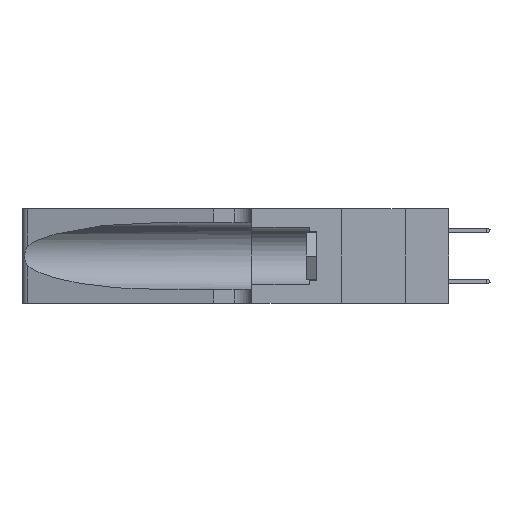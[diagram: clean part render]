
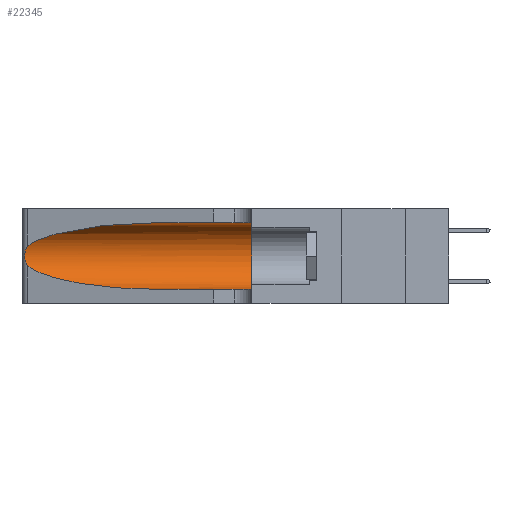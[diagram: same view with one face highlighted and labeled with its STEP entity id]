
A CAD part, left-side view. The second image highlights one B-rep face of the part: STEP entity #22345.
In plain terms, the highlighted cylindrical face has radius 3.308 mm (diameter 6.617 mm), a partial arc.
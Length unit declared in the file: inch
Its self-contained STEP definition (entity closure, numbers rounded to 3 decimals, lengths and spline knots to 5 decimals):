
#744 = CIRCLE ( 'NONE', #11254, 0.13025 ) ;
#951 = CARTESIAN_POINT ( 'NONE',  ( 0.1305, 0.35, 0.31525 ) ) ;
#1829 = ORIENTED_EDGE ( 'NONE', *, *, #18322, .F. ) ;
#2564 = CARTESIAN_POINT ( 'NONE',  ( 0.26017, 1.23833, 0.17102 ) ) ;
#2788 = LINE ( 'NONE', #3712, #29474 ) ;
#2856 = ORIENTED_EDGE ( 'NONE', *, *, #6467, .T. ) ;
#3712 = CARTESIAN_POINT ( 'NONE',  ( 0.1305, 1.61858, 0.05475 ) ) ;
#3921 = CARTESIAN_POINT ( 'NONE',  ( 0.26075, 1.23896, 0.19203 ) ) ;
#4350 = VERTEX_POINT ( 'NONE', #24508 ) ;
#4624 = B_SPLINE_CURVE_WITH_KNOTS ( 'NONE', 3,
 ( #23234, #12835, #28358, #12942, #30916, #15528, #3921, #18099, #2564, #20716, #5181, #23336, #7820, #25904 ),
 .UNSPECIFIED., .F., .F.,
 ( 4, 2, 2, 2, 2, 2, 4 ),
 ( 0., 0.00027, 0.00053, 0.00107, 0.0016, 0.00187, 0.00214 ),
 .UNSPECIFIED. ) ;
#4976 = CARTESIAN_POINT ( 'NONE',  ( 0.1305, 0.35, 0.185 ) ) ;
#5181 = CARTESIAN_POINT ( 'NONE',  ( 0.25789, 1.23486, 0.15765 ) ) ;
#6467 = EDGE_CURVE ( 'NONE', #20797, #4350, #19176, .T. ) ;
#6964 = CARTESIAN_POINT ( 'NONE',  ( 0.18966, 0.96281, 0.31525 ) ) ;
#7266 = EDGE_LOOP ( 'NONE', ( #2856, #14822, #15873, #10875, #1829, #7326 ) ) ;
#7326 = ORIENTED_EDGE ( 'NONE', *, *, #24627, .F. ) ;
#7609 = DIRECTION ( 'NONE',  ( 0., 0., 1. ) ) ;
#7820 = CARTESIAN_POINT ( 'NONE',  ( 0.25555, 1.22993, 0.14849 ) ) ;
#7839 = DIRECTION ( 'NONE',  ( 0., 0., -1. ) ) ;
#8406 = CARTESIAN_POINT ( 'NONE',  ( 0.18966, 0.96281, 0.05475 ) ) ;
#9448 = VECTOR ( 'NONE', #11316, 39.37008 ) ;
#10678 =( BOUNDED_CURVE ( )  B_SPLINE_CURVE ( 3, ( #18705, #10918, #8406, #26484 ),
 .UNSPECIFIED., .F., .T. ) 
 B_SPLINE_CURVE_WITH_KNOTS ( ( 4, 4 ),
 ( 3.44316, 4.71239 ),
 .UNSPECIFIED. ) 
 CURVE ( )  GEOMETRIC_REPRESENTATION_ITEM ( )  RATIONAL_B_SPLINE_CURVE ( ( 1., 0.87, 0.87, 1. ) ) 
 REPRESENTATION_ITEM ( '' )  );
#10875 = ORIENTED_EDGE ( 'NONE', *, *, #18711, .T. ) ;
#10918 = CARTESIAN_POINT ( 'NONE',  ( 0.2373, 1.15595, 0.08982 ) ) ;
#11254 = AXIS2_PLACEMENT_3D ( 'NONE', #4976, #23130, #7609 ) ;
#11316 = DIRECTION ( 'NONE',  ( 0., -1., 0. ) ) ;
#11328 = VERTEX_POINT ( 'NONE', #19131 ) ;
#12050 = FACE_OUTER_BOUND ( 'NONE', #7266, .T. ) ;
#12204 = CARTESIAN_POINT ( 'NONE',  ( 0.25487, 1.22718, 0.22369 ) ) ;
#12835 = CARTESIAN_POINT ( 'NONE',  ( 0.25555, 1.22994, 0.2215 ) ) ;
#12942 = CARTESIAN_POINT ( 'NONE',  ( 0.25787, 1.23484, 0.2124 ) ) ;
#14822 = ORIENTED_EDGE ( 'NONE', *, *, #30106, .T. ) ;
#15528 = CARTESIAN_POINT ( 'NONE',  ( 0.26018, 1.23835, 0.19895 ) ) ;
#15544 = DIRECTION ( 'NONE',  ( 0., -1., 0. ) ) ;
#15873 = ORIENTED_EDGE ( 'NONE', *, *, #29612, .T. ) ;
#18099 = CARTESIAN_POINT ( 'NONE',  ( 0.26075, 1.23896, 0.178 ) ) ;
#18322 = EDGE_CURVE ( 'NONE', #29056, #11328, #744, .T. ) ;
#18705 = CARTESIAN_POINT ( 'NONE',  ( 0.25487, 1.22718, 0.14631 ) ) ;
#18711 = EDGE_CURVE ( 'NONE', #31708, #11328, #2788, .T. ) ;
#18975 = CARTESIAN_POINT ( 'NONE',  ( 0.1305, 1.61858, 0.31525 ) ) ;
#19131 = CARTESIAN_POINT ( 'NONE',  ( 0.1305, 0.35, 0.05475 ) ) ;
#19176 =( BOUNDED_CURVE ( )  B_SPLINE_CURVE ( 3, ( #22364, #6964, #27633, #12204 ),
 .UNSPECIFIED., .F., .F. ) 
 B_SPLINE_CURVE_WITH_KNOTS ( ( 4, 4 ),
 ( 1.5708, 2.84003 ),
 .UNSPECIFIED. ) 
 CURVE ( )  GEOMETRIC_REPRESENTATION_ITEM ( )  RATIONAL_B_SPLINE_CURVE ( ( 1., 0.87, 0.87, 1. ) ) 
 REPRESENTATION_ITEM ( '' )  );
#20716 = CARTESIAN_POINT ( 'NONE',  ( 0.25856, 1.23593, 0.16098 ) ) ;
#20797 = VERTEX_POINT ( 'NONE', #22776 ) ;
#22345 = ADVANCED_FACE ( 'NONE', ( #12050 ), #24975, .F. ) ;
#22364 = CARTESIAN_POINT ( 'NONE',  ( 0.1305, 0.72297, 0.31525 ) ) ;
#22589 = VERTEX_POINT ( 'NONE', #24348 ) ;
#22776 = CARTESIAN_POINT ( 'NONE',  ( 0.1305, 0.72297, 0.31525 ) ) ;
#23130 = DIRECTION ( 'NONE',  ( 0., 1., 0. ) ) ;
#23234 = CARTESIAN_POINT ( 'NONE',  ( 0.25487, 1.22718, 0.22369 ) ) ;
#23336 = CARTESIAN_POINT ( 'NONE',  ( 0.25639, 1.23186, 0.15144 ) ) ;
#24348 = CARTESIAN_POINT ( 'NONE',  ( 0.25487, 1.22718, 0.14631 ) ) ;
#24508 = CARTESIAN_POINT ( 'NONE',  ( 0.25487, 1.22718, 0.22369 ) ) ;
#24627 = EDGE_CURVE ( 'NONE', #20797, #29056, #29988, .T. ) ;
#24937 = CARTESIAN_POINT ( 'NONE',  ( 0.1305, 0.72297, 0.05475 ) ) ;
#24975 = CYLINDRICAL_SURFACE ( 'NONE', #26660, 0.13025 ) ;
#25904 = CARTESIAN_POINT ( 'NONE',  ( 0.25487, 1.22718, 0.14631 ) ) ;
#26484 = CARTESIAN_POINT ( 'NONE',  ( 0.1305, 0.72297, 0.05475 ) ) ;
#26660 = AXIS2_PLACEMENT_3D ( 'NONE', #28476, #15544, #7839 ) ;
#27022 = DIRECTION ( 'NONE',  ( 0., -1., 0. ) ) ;
#27633 = CARTESIAN_POINT ( 'NONE',  ( 0.2373, 1.15595, 0.28018 ) ) ;
#28358 = CARTESIAN_POINT ( 'NONE',  ( 0.25639, 1.23184, 0.21858 ) ) ;
#28476 = CARTESIAN_POINT ( 'NONE',  ( 0.1305, 1.61858, 0.185 ) ) ;
#29056 = VERTEX_POINT ( 'NONE', #951 ) ;
#29474 = VECTOR ( 'NONE', #27022, 39.37008 ) ;
#29612 = EDGE_CURVE ( 'NONE', #22589, #31708, #10678, .T. ) ;
#29988 = LINE ( 'NONE', #18975, #9448 ) ;
#30106 = EDGE_CURVE ( 'NONE', #4350, #22589, #4624, .T. ) ;
#30916 = CARTESIAN_POINT ( 'NONE',  ( 0.25854, 1.2359, 0.20912 ) ) ;
#31708 = VERTEX_POINT ( 'NONE', #24937 ) ;
